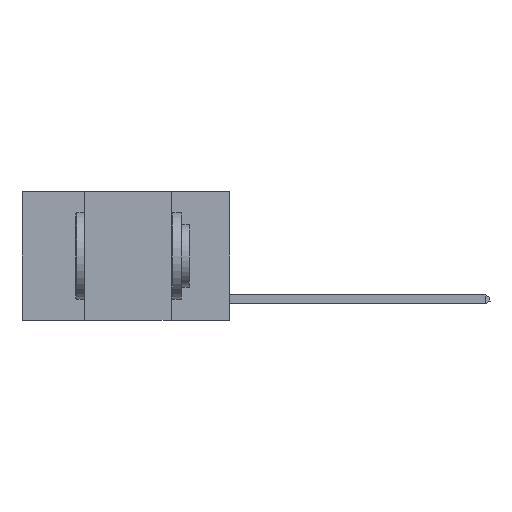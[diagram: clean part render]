
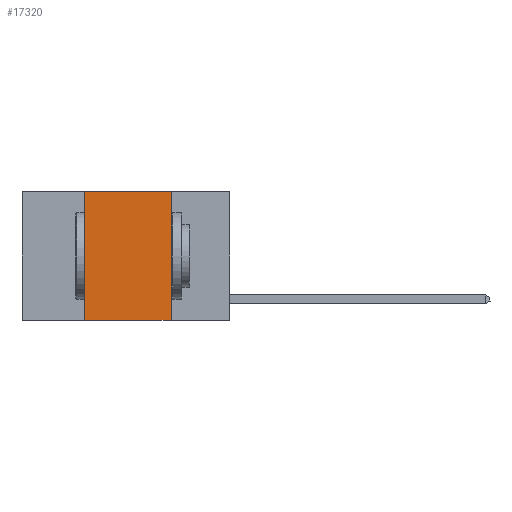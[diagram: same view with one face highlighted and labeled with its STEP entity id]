
A CAD part, left-side view. The second image highlights one B-rep face of the part: STEP entity #17320.
In plain terms, the highlighted planar face has unit normal (-1, 0, 0).
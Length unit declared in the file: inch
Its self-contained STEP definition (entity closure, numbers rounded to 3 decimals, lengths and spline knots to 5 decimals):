
#55 = ORIENTED_EDGE ( 'NONE', *, *, #19975, .F. ) ;
#493 = AXIS2_PLACEMENT_3D ( 'NONE', #18512, #7240, #20391 ) ;
#755 = LINE ( 'NONE', #13259, #19743 ) ;
#3396 = CARTESIAN_POINT ( 'NONE',  ( 0., 0.42, 0. ) ) ;
#3793 = DIRECTION ( 'NONE',  ( 0., 0., -1. ) ) ;
#3976 = CARTESIAN_POINT ( 'NONE',  ( 0., 0.42, 0. ) ) ;
#4135 = VERTEX_POINT ( 'NONE', #3976 ) ;
#5323 = PLANE ( 'NONE',  #493 ) ;
#5344 = DIRECTION ( 'NONE',  ( 0., 0., 1. ) ) ;
#5969 = EDGE_CURVE ( 'NONE', #4135, #10405, #19002, .T. ) ;
#7240 = DIRECTION ( 'NONE',  ( 1., 0., 0. ) ) ;
#8474 = ORIENTED_EDGE ( 'NONE', *, *, #5969, .F. ) ;
#9125 = ORIENTED_EDGE ( 'NONE', *, *, #17482, .F. ) ;
#9462 = VECTOR ( 'NONE', #5344, 39.37008 ) ;
#10405 = VERTEX_POINT ( 'NONE', #19224 ) ;
#11047 = LINE ( 'NONE', #17212, #20407 ) ;
#11593 = VERTEX_POINT ( 'NONE', #12782 ) ;
#12782 = CARTESIAN_POINT ( 'NONE',  ( 0., 0.17, -0.37 ) ) ;
#13259 = CARTESIAN_POINT ( 'NONE',  ( 0., 0.17, 0. ) ) ;
#14971 = EDGE_CURVE ( 'NONE', #21883, #11593, #11047, .T. ) ;
#14989 = ORIENTED_EDGE ( 'NONE', *, *, #14971, .T. ) ;
#17212 = CARTESIAN_POINT ( 'NONE',  ( 0., 0.6, -0.37 ) ) ;
#17320 = ADVANCED_FACE ( 'NONE', ( #19720 ), #5323, .F. ) ;
#17482 = EDGE_CURVE ( 'NONE', #21883, #4135, #24301, .T. ) ;
#17874 = CARTESIAN_POINT ( 'NONE',  ( 0., 0.42, -0.37 ) ) ;
#18418 = VECTOR ( 'NONE', #21453, 39.37008 ) ;
#18512 = CARTESIAN_POINT ( 'NONE',  ( 0., 0.6, 0. ) ) ;
#19002 = LINE ( 'NONE', #23206, #18418 ) ;
#19104 = DIRECTION ( 'NONE',  ( 0., -1., 0. ) ) ;
#19224 = CARTESIAN_POINT ( 'NONE',  ( 0., 0.17, 0. ) ) ;
#19720 = FACE_OUTER_BOUND ( 'NONE', #23601, .T. ) ;
#19743 = VECTOR ( 'NONE', #3793, 39.37008 ) ;
#19975 = EDGE_CURVE ( 'NONE', #10405, #11593, #755, .T. ) ;
#20391 = DIRECTION ( 'NONE',  ( 0., 0., -1. ) ) ;
#20407 = VECTOR ( 'NONE', #19104, 39.37008 ) ;
#21453 = DIRECTION ( 'NONE',  ( 0., -1., 0. ) ) ;
#21883 = VERTEX_POINT ( 'NONE', #17874 ) ;
#23206 = CARTESIAN_POINT ( 'NONE',  ( 0., 0.6, 0. ) ) ;
#23601 = EDGE_LOOP ( 'NONE', ( #55, #8474, #9125, #14989 ) ) ;
#24301 = LINE ( 'NONE', #3396, #9462 ) ;
